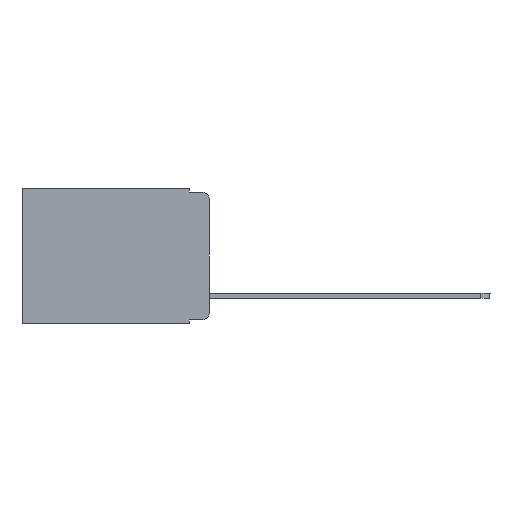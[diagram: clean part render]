
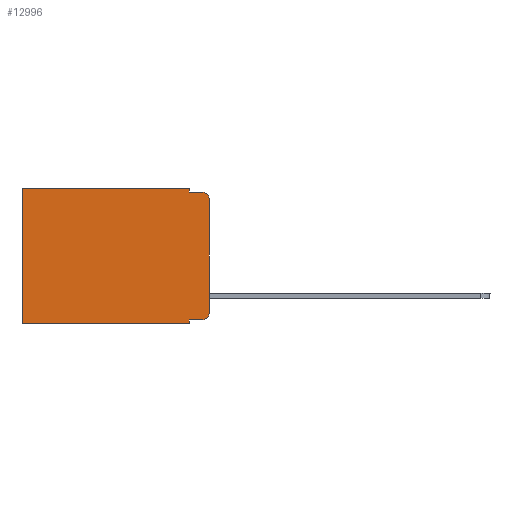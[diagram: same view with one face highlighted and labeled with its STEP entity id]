
A CAD part, left-side view. The second image highlights one B-rep face of the part: STEP entity #12996.
In plain terms, the highlighted planar face has unit normal (-1, 0, 0).
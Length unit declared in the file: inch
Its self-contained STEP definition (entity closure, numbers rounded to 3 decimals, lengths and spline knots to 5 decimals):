
#41 = VERTEX_POINT ( 'NONE', #3825 ) ;
#633 = CARTESIAN_POINT ( 'NONE',  ( 0.298, 0., -0.03 ) ) ;
#732 = LINE ( 'NONE', #10090, #8539 ) ;
#890 = DIRECTION ( 'NONE',  ( -1., 0., 0. ) ) ;
#980 = CARTESIAN_POINT ( 'NONE',  ( 0.298, 0.02, -0.03 ) ) ;
#1159 = EDGE_CURVE ( 'NONE', #41, #12577, #3527, .T. ) ;
#1164 = DIRECTION ( 'NONE',  ( 0., 0., -1. ) ) ;
#1300 = CARTESIAN_POINT ( 'NONE',  ( 0.298, 0.473, 0. ) ) ;
#1630 = VERTEX_POINT ( 'NONE', #8025 ) ;
#1676 = EDGE_CURVE ( 'NONE', #1815, #4751, #15157, .T. ) ;
#1815 = VERTEX_POINT ( 'NONE', #9713 ) ;
#2200 = CARTESIAN_POINT ( 'NONE',  ( 0.298, 0., 0. ) ) ;
#2278 = PLANE ( 'NONE',  #6779 ) ;
#2374 = ORIENTED_EDGE ( 'NONE', *, *, #1676, .F. ) ;
#2380 = CARTESIAN_POINT ( 'NONE',  ( 0.298, 0., 0. ) ) ;
#2429 = FACE_OUTER_BOUND ( 'NONE', #14039, .T. ) ;
#2477 = CARTESIAN_POINT ( 'NONE',  ( 0.298, 0.051, 0. ) ) ;
#2865 = LINE ( 'NONE', #10844, #7841 ) ;
#3060 = LINE ( 'NONE', #13410, #12172 ) ;
#3088 = VECTOR ( 'NONE', #12866, 39.37008 ) ;
#3162 = CIRCLE ( 'NONE', #9526, 0.02 ) ;
#3203 = EDGE_CURVE ( 'NONE', #6186, #1815, #3398, .T. ) ;
#3398 = LINE ( 'NONE', #7157, #10976 ) ;
#3527 = LINE ( 'NONE', #1300, #3088 ) ;
#3606 = CARTESIAN_POINT ( 'NONE',  ( 0.298, 0.02, -0.01 ) ) ;
#3825 = CARTESIAN_POINT ( 'NONE',  ( 0.298, 0.473, 0. ) ) ;
#3979 = CARTESIAN_POINT ( 'NONE',  ( 0.298, 0.051, -0.333 ) ) ;
#4331 = EDGE_CURVE ( 'NONE', #1630, #5360, #14917, .T. ) ;
#4719 = CARTESIAN_POINT ( 'NONE',  ( 0.298, 0.051, -0.343 ) ) ;
#4751 = VERTEX_POINT ( 'NONE', #3606 ) ;
#4818 = ORIENTED_EDGE ( 'NONE', *, *, #7423, .F. ) ;
#4823 = ORIENTED_EDGE ( 'NONE', *, *, #12179, .T. ) ;
#4878 = DIRECTION ( 'NONE',  ( 0., -1., 0. ) ) ;
#5101 = ORIENTED_EDGE ( 'NONE', *, *, #14904, .T. ) ;
#5273 = LINE ( 'NONE', #3979, #9842 ) ;
#5360 = VERTEX_POINT ( 'NONE', #11248 ) ;
#5536 = ORIENTED_EDGE ( 'NONE', *, *, #1159, .T. ) ;
#5657 = DIRECTION ( 'NONE',  ( -1., 0., 0. ) ) ;
#5691 = DIRECTION ( 'NONE',  ( 0., 1., 0. ) ) ;
#6186 = VERTEX_POINT ( 'NONE', #2477 ) ;
#6439 = EDGE_CURVE ( 'NONE', #12523, #4751, #3162, .T. ) ;
#6779 = AXIS2_PLACEMENT_3D ( 'NONE', #2200, #8115, #11561 ) ;
#6790 = AXIS2_PLACEMENT_3D ( 'NONE', #13781, #890, #13845 ) ;
#7157 = CARTESIAN_POINT ( 'NONE',  ( 0.298, 0.051, 0. ) ) ;
#7423 = EDGE_CURVE ( 'NONE', #12523, #5360, #732, .T. ) ;
#7554 = VECTOR ( 'NONE', #4878, 39.37008 ) ;
#7741 = DIRECTION ( 'NONE',  ( 0., 0., -1. ) ) ;
#7841 = VECTOR ( 'NONE', #14457, 39.37008 ) ;
#7896 = DIRECTION ( 'NONE',  ( 0., 0., -1. ) ) ;
#7915 = ORIENTED_EDGE ( 'NONE', *, *, #4331, .T. ) ;
#8025 = CARTESIAN_POINT ( 'NONE',  ( 0.298, 0.02, -0.333 ) ) ;
#8105 = VECTOR ( 'NONE', #5691, 39.37008 ) ;
#8115 = DIRECTION ( 'NONE',  ( 1., 0., 0. ) ) ;
#8338 = CARTESIAN_POINT ( 'NONE',  ( 0.298, 0.051, -0.01 ) ) ;
#8539 = VECTOR ( 'NONE', #14768, 39.37008 ) ;
#9526 = AXIS2_PLACEMENT_3D ( 'NONE', #980, #5657, #7896 ) ;
#9649 = ORIENTED_EDGE ( 'NONE', *, *, #12960, .F. ) ;
#9686 = VERTEX_POINT ( 'NONE', #4719 ) ;
#9713 = CARTESIAN_POINT ( 'NONE',  ( 0.298, 0.051, -0.01 ) ) ;
#9842 = VECTOR ( 'NONE', #13566, 39.37008 ) ;
#10090 = CARTESIAN_POINT ( 'NONE',  ( 0.298, 0., 0. ) ) ;
#10218 = CARTESIAN_POINT ( 'NONE',  ( 0.298, 0.051, -0.333 ) ) ;
#10590 = EDGE_CURVE ( 'NONE', #9686, #12577, #2865, .T. ) ;
#10767 = VERTEX_POINT ( 'NONE', #10218 ) ;
#10844 = CARTESIAN_POINT ( 'NONE',  ( 0.298, 0., -0.343 ) ) ;
#10976 = VECTOR ( 'NONE', #1164, 39.37008 ) ;
#11248 = CARTESIAN_POINT ( 'NONE',  ( 0.298, 0., -0.313 ) ) ;
#11394 = ORIENTED_EDGE ( 'NONE', *, *, #3203, .F. ) ;
#11561 = DIRECTION ( 'NONE',  ( 0., 0., -1. ) ) ;
#11749 = LINE ( 'NONE', #2380, #8105 ) ;
#12172 = VECTOR ( 'NONE', #7741, 39.37008 ) ;
#12179 = EDGE_CURVE ( 'NONE', #6186, #41, #11749, .T. ) ;
#12523 = VERTEX_POINT ( 'NONE', #633 ) ;
#12577 = VERTEX_POINT ( 'NONE', #12800 ) ;
#12800 = CARTESIAN_POINT ( 'NONE',  ( 0.298, 0.473, -0.343 ) ) ;
#12866 = DIRECTION ( 'NONE',  ( 0., 0., -1. ) ) ;
#12960 = EDGE_CURVE ( 'NONE', #10767, #9686, #3060, .T. ) ;
#12996 = ADVANCED_FACE ( 'NONE', ( #2429 ), #2278, .F. ) ;
#13410 = CARTESIAN_POINT ( 'NONE',  ( 0.298, 0.051, 0. ) ) ;
#13566 = DIRECTION ( 'NONE',  ( 0., -1., 0. ) ) ;
#13781 = CARTESIAN_POINT ( 'NONE',  ( 0.298, 0.02, -0.313 ) ) ;
#13845 = DIRECTION ( 'NONE',  ( 0., 0., -1. ) ) ;
#14039 = EDGE_LOOP ( 'NONE', ( #4818, #14627, #2374, #11394, #4823, #5536, #14825, #9649, #5101, #7915 ) ) ;
#14457 = DIRECTION ( 'NONE',  ( 0., 1., 0. ) ) ;
#14627 = ORIENTED_EDGE ( 'NONE', *, *, #6439, .T. ) ;
#14768 = DIRECTION ( 'NONE',  ( 0., 0., -1. ) ) ;
#14825 = ORIENTED_EDGE ( 'NONE', *, *, #10590, .F. ) ;
#14904 = EDGE_CURVE ( 'NONE', #10767, #1630, #5273, .T. ) ;
#14917 = CIRCLE ( 'NONE', #6790, 0.02 ) ;
#15157 = LINE ( 'NONE', #8338, #7554 ) ;
